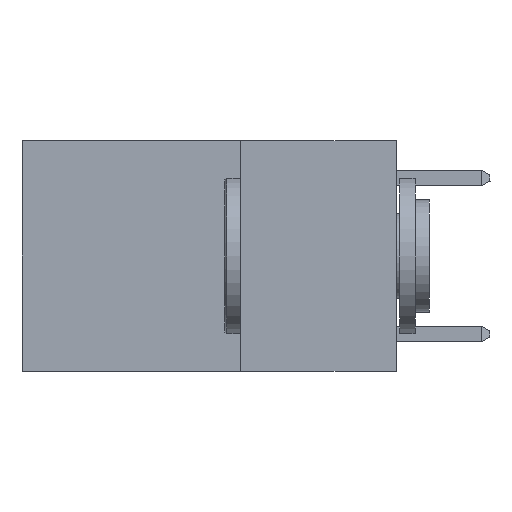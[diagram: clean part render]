
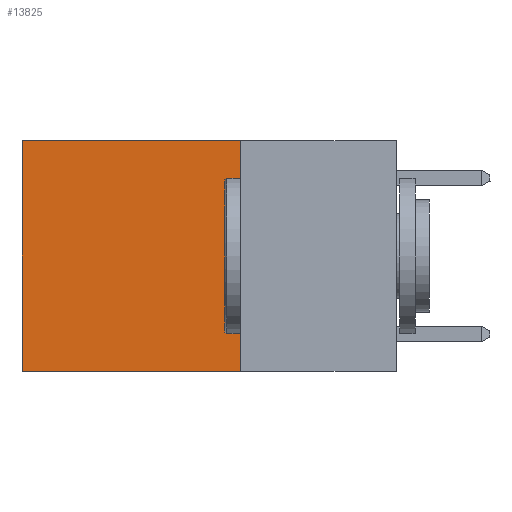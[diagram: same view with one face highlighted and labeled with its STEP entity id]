
A CAD part, left-side view. The second image highlights one B-rep face of the part: STEP entity #13825.
In plain terms, the highlighted planar face has unit normal (-1, 0, 0).
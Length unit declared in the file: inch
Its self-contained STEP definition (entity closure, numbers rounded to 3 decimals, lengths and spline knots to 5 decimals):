
#3159 = VECTOR ( 'NONE', #18158, 39.37008 ) ;
#3831 = ORIENTED_EDGE ( 'NONE', *, *, #6962, .T. ) ;
#4028 = VECTOR ( 'NONE', #13067, 39.37008 ) ;
#4101 = ORIENTED_EDGE ( 'NONE', *, *, #22586, .T. ) ;
#5102 = DIRECTION ( 'NONE',  ( 1., 0., 0. ) ) ;
#6962 = EDGE_CURVE ( 'NONE', #25755, #12802, #14055, .T. ) ;
#7602 = VECTOR ( 'NONE', #15270, 39.37008 ) ;
#8380 = CARTESIAN_POINT ( 'NONE',  ( 0.2625, 0.25, 0. ) ) ;
#8630 = CARTESIAN_POINT ( 'NONE',  ( 0.2625, 0.6, 0. ) ) ;
#8669 = LINE ( 'NONE', #8380, #4028 ) ;
#9129 = AXIS2_PLACEMENT_3D ( 'NONE', #17873, #5102, #22029 ) ;
#9235 = CARTESIAN_POINT ( 'NONE',  ( 0.2625, 0.25, 0. ) ) ;
#12802 = VERTEX_POINT ( 'NONE', #8630 ) ;
#13067 = DIRECTION ( 'NONE',  ( 0., 0., -1. ) ) ;
#13211 = CARTESIAN_POINT ( 'NONE',  ( 0.2625, 0.6, -0.37 ) ) ;
#13825 = ADVANCED_FACE ( 'NONE', ( #24587 ), #24450, .F. ) ;
#14055 = LINE ( 'NONE', #18012, #3159 ) ;
#15146 = ORIENTED_EDGE ( 'NONE', *, *, #22844, .F. ) ;
#15270 = DIRECTION ( 'NONE',  ( 0., 1., 0. ) ) ;
#15659 = VERTEX_POINT ( 'NONE', #13211 ) ;
#16012 = CARTESIAN_POINT ( 'NONE',  ( 0.2625, 0.25, -0.37 ) ) ;
#17474 = CARTESIAN_POINT ( 'NONE',  ( 0.2625, 0.25, -0.37 ) ) ;
#17873 = CARTESIAN_POINT ( 'NONE',  ( 0.2625, 0.25, 0. ) ) ;
#18001 = LINE ( 'NONE', #22422, #23019 ) ;
#18012 = CARTESIAN_POINT ( 'NONE',  ( 0.2625, 0.25, 0. ) ) ;
#18158 = DIRECTION ( 'NONE',  ( 0., 1., 0. ) ) ;
#19824 = EDGE_LOOP ( 'NONE', ( #4101, #15146, #24541, #3831 ) ) ;
#20290 = VERTEX_POINT ( 'NONE', #17474 ) ;
#22029 = DIRECTION ( 'NONE',  ( 0., 0., -1. ) ) ;
#22422 = CARTESIAN_POINT ( 'NONE',  ( 0.2625, 0.6, 0. ) ) ;
#22586 = EDGE_CURVE ( 'NONE', #12802, #15659, #18001, .T. ) ;
#22844 = EDGE_CURVE ( 'NONE', #20290, #15659, #26836, .T. ) ;
#23019 = VECTOR ( 'NONE', #24294, 39.37008 ) ;
#24167 = EDGE_CURVE ( 'NONE', #25755, #20290, #8669, .T. ) ;
#24294 = DIRECTION ( 'NONE',  ( 0., 0., -1. ) ) ;
#24450 = PLANE ( 'NONE',  #9129 ) ;
#24541 = ORIENTED_EDGE ( 'NONE', *, *, #24167, .F. ) ;
#24587 = FACE_OUTER_BOUND ( 'NONE', #19824, .T. ) ;
#25755 = VERTEX_POINT ( 'NONE', #9235 ) ;
#26836 = LINE ( 'NONE', #16012, #7602 ) ;
